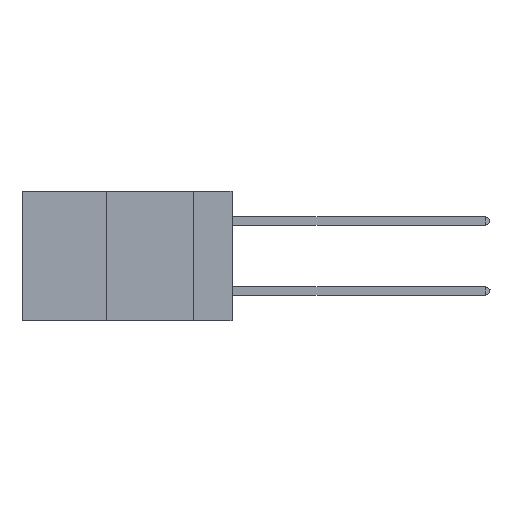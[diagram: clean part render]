
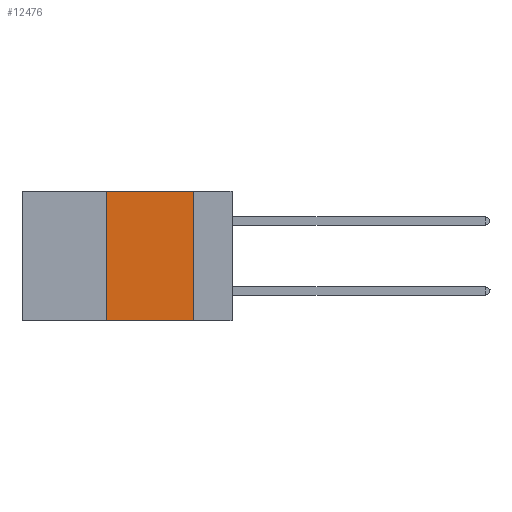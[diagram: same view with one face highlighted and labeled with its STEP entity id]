
A CAD part, left-side view. The second image highlights one B-rep face of the part: STEP entity #12476.
In plain terms, the highlighted planar face has unit normal (-1, 0, 0).
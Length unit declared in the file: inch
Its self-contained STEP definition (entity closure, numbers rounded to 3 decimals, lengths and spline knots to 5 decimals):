
#431 = EDGE_CURVE ( 'NONE', #25039, #23397, #3518, .T. ) ;
#845 = CARTESIAN_POINT ( 'NONE',  ( 0., 0.11, -0.37 ) ) ;
#2405 = CARTESIAN_POINT ( 'NONE',  ( 0., 0.6, 0. ) ) ;
#2800 = LINE ( 'NONE', #15894, #17726 ) ;
#2964 = DIRECTION ( 'NONE',  ( 0., 0., 1. ) ) ;
#3457 = CARTESIAN_POINT ( 'NONE',  ( 0., 0.6, -0.37 ) ) ;
#3518 = LINE ( 'NONE', #19159, #19106 ) ;
#7024 = CARTESIAN_POINT ( 'NONE',  ( 0., 0.6, 0. ) ) ;
#7715 = DIRECTION ( 'NONE',  ( 0., -1., 0. ) ) ;
#10096 = LINE ( 'NONE', #7024, #28489 ) ;
#11952 = EDGE_CURVE ( 'NONE', #20198, #25039, #10096, .T. ) ;
#12445 = DIRECTION ( 'NONE',  ( 1., 0., 0. ) ) ;
#12476 = ADVANCED_FACE ( 'NONE', ( #25520 ), #22967, .F. ) ;
#13056 = CARTESIAN_POINT ( 'NONE',  ( 0., 0.11, 0. ) ) ;
#13334 = AXIS2_PLACEMENT_3D ( 'NONE', #2405, #12445, #33335 ) ;
#14226 = DIRECTION ( 'NONE',  ( 0., 0., -1. ) ) ;
#15894 = CARTESIAN_POINT ( 'NONE',  ( 0., 0.36, 0. ) ) ;
#16596 = CARTESIAN_POINT ( 'NONE',  ( 0., 0.36, -0.37 ) ) ;
#17726 = VECTOR ( 'NONE', #2964, 39.37008 ) ;
#18706 = EDGE_CURVE ( 'NONE', #25357, #20198, #2800, .T. ) ;
#18915 = EDGE_CURVE ( 'NONE', #25357, #23397, #24363, .T. ) ;
#19062 = ORIENTED_EDGE ( 'NONE', *, *, #18915, .T. ) ;
#19106 = VECTOR ( 'NONE', #14226, 39.37008 ) ;
#19159 = CARTESIAN_POINT ( 'NONE',  ( 0., 0.11, 0. ) ) ;
#19431 = DIRECTION ( 'NONE',  ( 0., -1., 0. ) ) ;
#20198 = VERTEX_POINT ( 'NONE', #29643 ) ;
#21833 = ORIENTED_EDGE ( 'NONE', *, *, #431, .F. ) ;
#22075 = VECTOR ( 'NONE', #19431, 39.37008 ) ;
#22655 = ORIENTED_EDGE ( 'NONE', *, *, #18706, .F. ) ;
#22967 = PLANE ( 'NONE',  #13334 ) ;
#23397 = VERTEX_POINT ( 'NONE', #845 ) ;
#23585 = ORIENTED_EDGE ( 'NONE', *, *, #11952, .F. ) ;
#24363 = LINE ( 'NONE', #3457, #22075 ) ;
#25039 = VERTEX_POINT ( 'NONE', #13056 ) ;
#25357 = VERTEX_POINT ( 'NONE', #16596 ) ;
#25520 = FACE_OUTER_BOUND ( 'NONE', #29152, .T. ) ;
#28489 = VECTOR ( 'NONE', #7715, 39.37008 ) ;
#29152 = EDGE_LOOP ( 'NONE', ( #21833, #23585, #22655, #19062 ) ) ;
#29643 = CARTESIAN_POINT ( 'NONE',  ( 0., 0.36, 0. ) ) ;
#33335 = DIRECTION ( 'NONE',  ( 0., 0., -1. ) ) ;
